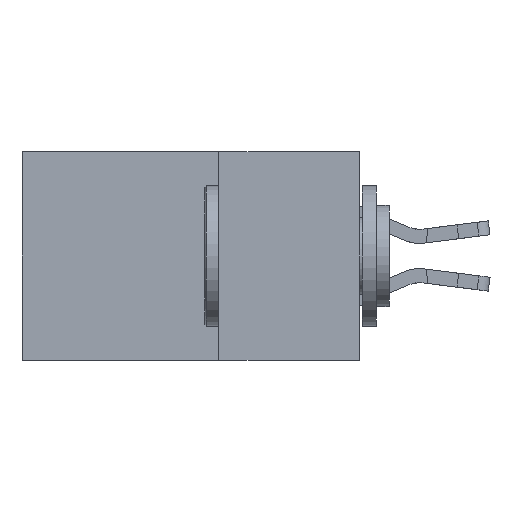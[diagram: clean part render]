
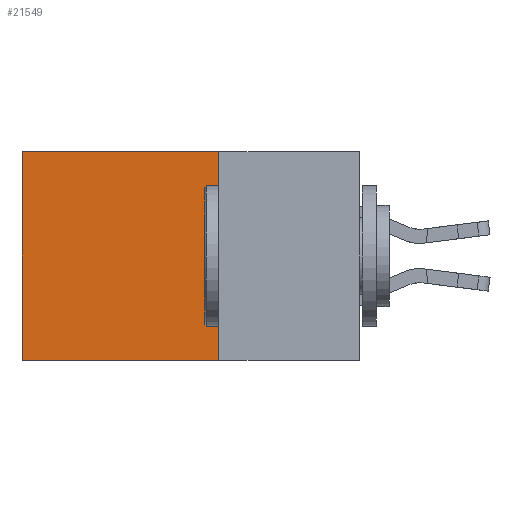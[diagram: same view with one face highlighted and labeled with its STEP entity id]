
A CAD part, left-side view. The second image highlights one B-rep face of the part: STEP entity #21549.
In plain terms, the highlighted planar face has unit normal (-1, 0, 0).
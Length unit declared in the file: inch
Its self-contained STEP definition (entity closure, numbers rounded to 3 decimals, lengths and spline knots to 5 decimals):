
#678 = VECTOR ( 'NONE', #3596, 39.37008 ) ;
#1967 = CARTESIAN_POINT ( 'NONE',  ( 0.2875, 0.25, 0. ) ) ;
#3013 = LINE ( 'NONE', #6320, #25608 ) ;
#3214 = ORIENTED_EDGE ( 'NONE', *, *, #16304, .T. ) ;
#3596 = DIRECTION ( 'NONE',  ( 0., 1., 0. ) ) ;
#3616 = AXIS2_PLACEMENT_3D ( 'NONE', #7291, #13879, #26409 ) ;
#3771 = CARTESIAN_POINT ( 'NONE',  ( 0.2875, 0.25, 0. ) ) ;
#4320 = VECTOR ( 'NONE', #23128, 39.37008 ) ;
#4714 = EDGE_CURVE ( 'NONE', #25870, #24282, #3013, .T. ) ;
#5450 = PLANE ( 'NONE',  #3616 ) ;
#6320 = CARTESIAN_POINT ( 'NONE',  ( 0.2875, 0.6, 0. ) ) ;
#7291 = CARTESIAN_POINT ( 'NONE',  ( 0.2875, 0.25, 0. ) ) ;
#7971 = VERTEX_POINT ( 'NONE', #12441 ) ;
#8036 = ORIENTED_EDGE ( 'NONE', *, *, #8416, .F. ) ;
#8095 = EDGE_LOOP ( 'NONE', ( #24632, #8036, #20510, #3214 ) ) ;
#8416 = EDGE_CURVE ( 'NONE', #7971, #24282, #11591, .T. ) ;
#10289 = CARTESIAN_POINT ( 'NONE',  ( 0.2875, 0.25, -0.37 ) ) ;
#10336 = DIRECTION ( 'NONE',  ( 0., 0., -1. ) ) ;
#11385 = EDGE_CURVE ( 'NONE', #20775, #7971, #13424, .T. ) ;
#11591 = LINE ( 'NONE', #10289, #678 ) ;
#12441 = CARTESIAN_POINT ( 'NONE',  ( 0.2875, 0.25, -0.37 ) ) ;
#12992 = CARTESIAN_POINT ( 'NONE',  ( 0.2875, 0.25, 0. ) ) ;
#13424 = LINE ( 'NONE', #3771, #14087 ) ;
#13879 = DIRECTION ( 'NONE',  ( 1., 0., 0. ) ) ;
#14087 = VECTOR ( 'NONE', #17139, 39.37008 ) ;
#16304 = EDGE_CURVE ( 'NONE', #20775, #25870, #26929, .T. ) ;
#17139 = DIRECTION ( 'NONE',  ( 0., 0., -1. ) ) ;
#20510 = ORIENTED_EDGE ( 'NONE', *, *, #11385, .F. ) ;
#20775 = VERTEX_POINT ( 'NONE', #12992 ) ;
#20866 = FACE_OUTER_BOUND ( 'NONE', #8095, .T. ) ;
#21549 = ADVANCED_FACE ( 'NONE', ( #20866 ), #5450, .F. ) ;
#23128 = DIRECTION ( 'NONE',  ( 0., 1., 0. ) ) ;
#24282 = VERTEX_POINT ( 'NONE', #25000 ) ;
#24632 = ORIENTED_EDGE ( 'NONE', *, *, #4714, .T. ) ;
#25000 = CARTESIAN_POINT ( 'NONE',  ( 0.2875, 0.6, -0.37 ) ) ;
#25608 = VECTOR ( 'NONE', #10336, 39.37008 ) ;
#25870 = VERTEX_POINT ( 'NONE', #26274 ) ;
#26274 = CARTESIAN_POINT ( 'NONE',  ( 0.2875, 0.6, 0. ) ) ;
#26409 = DIRECTION ( 'NONE',  ( 0., 0., -1. ) ) ;
#26929 = LINE ( 'NONE', #1967, #4320 ) ;
